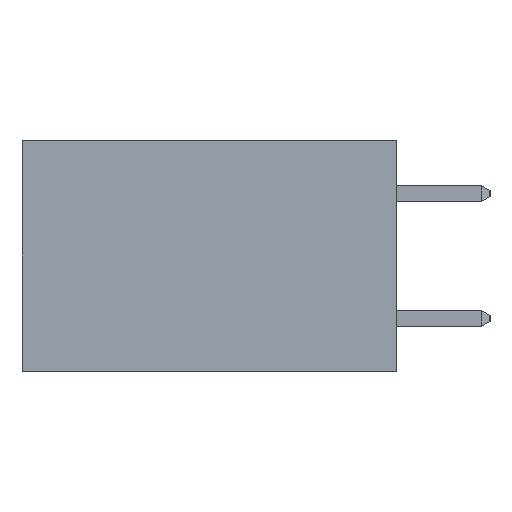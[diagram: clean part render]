
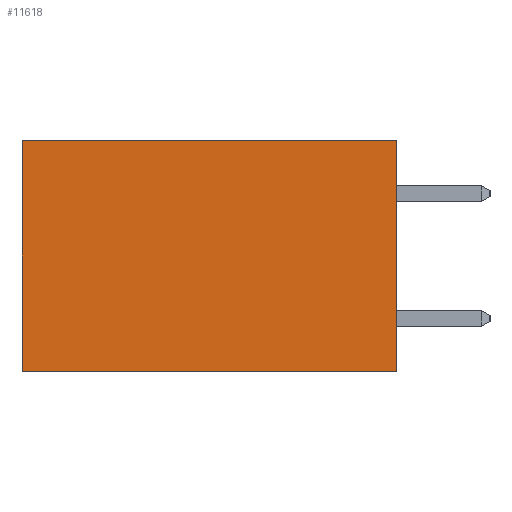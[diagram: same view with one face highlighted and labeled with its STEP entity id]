
A CAD part, left-side view. The second image highlights one B-rep face of the part: STEP entity #11618.
In plain terms, the highlighted planar face has unit normal (-1, 0, 0).
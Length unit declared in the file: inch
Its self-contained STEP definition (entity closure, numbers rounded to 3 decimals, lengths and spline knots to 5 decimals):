
#575 = LINE ( 'NONE', #18226, #16603 ) ;
#1105 = EDGE_CURVE ( 'NONE', #19251, #4003, #17752, .T. ) ;
#1499 = DIRECTION ( 'NONE',  ( 0., 0., -1. ) ) ;
#1981 = EDGE_CURVE ( 'NONE', #13698, #19021, #21848, .T. ) ;
#3104 = ORIENTED_EDGE ( 'NONE', *, *, #1981, .T. ) ;
#3528 = CARTESIAN_POINT ( 'NONE',  ( 0.298, 0.6, 0. ) ) ;
#4003 = VERTEX_POINT ( 'NONE', #14200 ) ;
#4500 = CARTESIAN_POINT ( 'NONE',  ( 0.298, 0., 0. ) ) ;
#4667 = LINE ( 'NONE', #3528, #25260 ) ;
#5628 = ORIENTED_EDGE ( 'NONE', *, *, #14406, .F. ) ;
#6065 = EDGE_LOOP ( 'NONE', ( #13291, #14958, #5628, #3104 ) ) ;
#6173 = CARTESIAN_POINT ( 'NONE',  ( 0.298, 0.6, 0. ) ) ;
#6202 = DIRECTION ( 'NONE',  ( 1., 0., 0. ) ) ;
#6264 = CARTESIAN_POINT ( 'NONE',  ( 0.298, 0., -0.37 ) ) ;
#8149 = CARTESIAN_POINT ( 'NONE',  ( 0.298, 0., 0. ) ) ;
#11618 = ADVANCED_FACE ( 'NONE', ( #21526 ), #14215, .F. ) ;
#13291 = ORIENTED_EDGE ( 'NONE', *, *, #24139, .T. ) ;
#13420 = DIRECTION ( 'NONE',  ( 0., 1., 0. ) ) ;
#13698 = VERTEX_POINT ( 'NONE', #8149 ) ;
#14200 = CARTESIAN_POINT ( 'NONE',  ( 0.298, 0.6, -0.37 ) ) ;
#14215 = PLANE ( 'NONE',  #18472 ) ;
#14406 = EDGE_CURVE ( 'NONE', #13698, #19251, #575, .T. ) ;
#14505 = DIRECTION ( 'NONE',  ( 0., 1., 0. ) ) ;
#14958 = ORIENTED_EDGE ( 'NONE', *, *, #1105, .F. ) ;
#16516 = VECTOR ( 'NONE', #13420, 39.37008 ) ;
#16603 = VECTOR ( 'NONE', #22075, 39.37008 ) ;
#17256 = VECTOR ( 'NONE', #14505, 39.37008 ) ;
#17752 = LINE ( 'NONE', #6264, #16516 ) ;
#18199 = CARTESIAN_POINT ( 'NONE',  ( 0.298, 0., 0. ) ) ;
#18226 = CARTESIAN_POINT ( 'NONE',  ( 0.298, 0., 0. ) ) ;
#18472 = AXIS2_PLACEMENT_3D ( 'NONE', #18199, #6202, #20158 ) ;
#19021 = VERTEX_POINT ( 'NONE', #6173 ) ;
#19251 = VERTEX_POINT ( 'NONE', #20194 ) ;
#20158 = DIRECTION ( 'NONE',  ( 0., 0., -1. ) ) ;
#20194 = CARTESIAN_POINT ( 'NONE',  ( 0.298, 0., -0.37 ) ) ;
#21526 = FACE_OUTER_BOUND ( 'NONE', #6065, .T. ) ;
#21848 = LINE ( 'NONE', #4500, #17256 ) ;
#22075 = DIRECTION ( 'NONE',  ( 0., 0., -1. ) ) ;
#24139 = EDGE_CURVE ( 'NONE', #19021, #4003, #4667, .T. ) ;
#25260 = VECTOR ( 'NONE', #1499, 39.37008 ) ;
